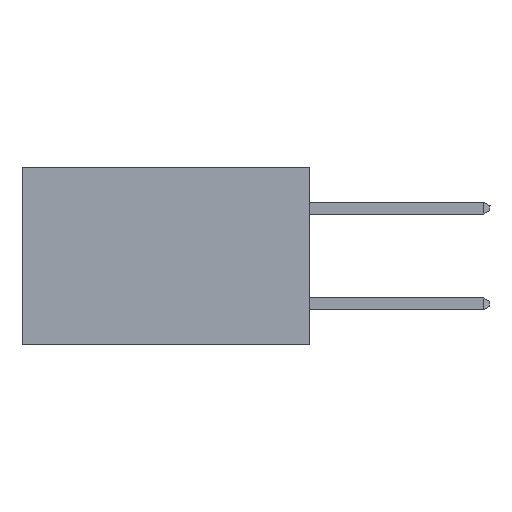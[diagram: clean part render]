
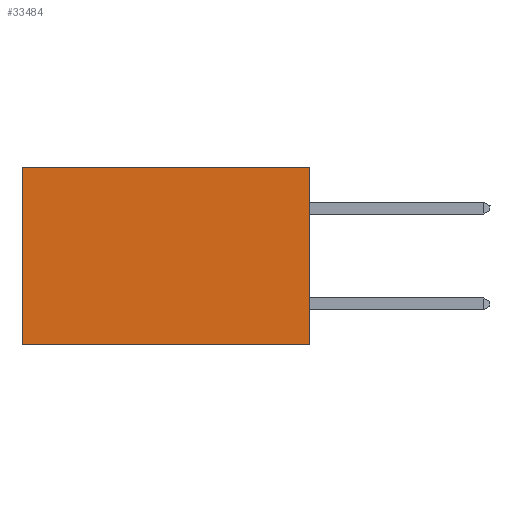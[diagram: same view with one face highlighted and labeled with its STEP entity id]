
A CAD part, left-side view. The second image highlights one B-rep face of the part: STEP entity #33484.
In plain terms, the highlighted planar face has unit normal (-1, 0, 0).
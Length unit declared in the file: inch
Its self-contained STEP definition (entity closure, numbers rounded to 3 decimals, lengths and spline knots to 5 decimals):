
#1404 = VERTEX_POINT ( 'NONE', #41994 ) ;
#2174 = CARTESIAN_POINT ( 'NONE',  ( 0.2875, 0., 0. ) ) ;
#4412 = AXIS2_PLACEMENT_3D ( 'NONE', #2174, #5763, #30470 ) ;
#4657 = VECTOR ( 'NONE', #10347, 39.37008 ) ;
#5763 = DIRECTION ( 'NONE',  ( 1., 0., 0. ) ) ;
#7022 = DIRECTION ( 'NONE',  ( 0., 0., -1. ) ) ;
#8778 = LINE ( 'NONE', #33521, #17073 ) ;
#8950 = LINE ( 'NONE', #33430, #17237 ) ;
#10347 = DIRECTION ( 'NONE',  ( 0., 0., -1. ) ) ;
#10600 = CARTESIAN_POINT ( 'NONE',  ( 0.2875, 0., 0. ) ) ;
#11394 = CARTESIAN_POINT ( 'NONE',  ( 0.2875, 0.6, -0.37 ) ) ;
#13646 = VECTOR ( 'NONE', #7022, 39.37008 ) ;
#14740 = LINE ( 'NONE', #10600, #13646 ) ;
#15839 = DIRECTION ( 'NONE',  ( 0., 1., 0. ) ) ;
#17073 = VECTOR ( 'NONE', #23053, 39.37008 ) ;
#17237 = VECTOR ( 'NONE', #15839, 39.37008 ) ;
#18124 = ORIENTED_EDGE ( 'NONE', *, *, #30339, .F. ) ;
#19108 = ORIENTED_EDGE ( 'NONE', *, *, #45327, .T. ) ;
#21516 = EDGE_CURVE ( 'NONE', #39990, #35153, #14740, .T. ) ;
#22456 = EDGE_LOOP ( 'NONE', ( #19108, #18124, #32039, #24395 ) ) ;
#23053 = DIRECTION ( 'NONE',  ( 0., 1., 0. ) ) ;
#24395 = ORIENTED_EDGE ( 'NONE', *, *, #43187, .T. ) ;
#25200 = FACE_OUTER_BOUND ( 'NONE', #22456, .T. ) ;
#30339 = EDGE_CURVE ( 'NONE', #35153, #40313, #8950, .T. ) ;
#30470 = DIRECTION ( 'NONE',  ( 0., 0., -1. ) ) ;
#32039 = ORIENTED_EDGE ( 'NONE', *, *, #21516, .F. ) ;
#33430 = CARTESIAN_POINT ( 'NONE',  ( 0.2875, 0., -0.37 ) ) ;
#33484 = ADVANCED_FACE ( 'NONE', ( #25200 ), #44433, .F. ) ;
#33521 = CARTESIAN_POINT ( 'NONE',  ( 0.2875, 0., 0. ) ) ;
#33773 = CARTESIAN_POINT ( 'NONE',  ( 0.2875, 0., 0. ) ) ;
#34285 = CARTESIAN_POINT ( 'NONE',  ( 0.2875, 0., -0.37 ) ) ;
#35029 = CARTESIAN_POINT ( 'NONE',  ( 0.2875, 0.6, 0. ) ) ;
#35153 = VERTEX_POINT ( 'NONE', #34285 ) ;
#39990 = VERTEX_POINT ( 'NONE', #33773 ) ;
#40313 = VERTEX_POINT ( 'NONE', #11394 ) ;
#41122 = LINE ( 'NONE', #35029, #4657 ) ;
#41994 = CARTESIAN_POINT ( 'NONE',  ( 0.2875, 0.6, 0. ) ) ;
#43187 = EDGE_CURVE ( 'NONE', #39990, #1404, #8778, .T. ) ;
#44433 = PLANE ( 'NONE',  #4412 ) ;
#45327 = EDGE_CURVE ( 'NONE', #1404, #40313, #41122, .T. ) ;
